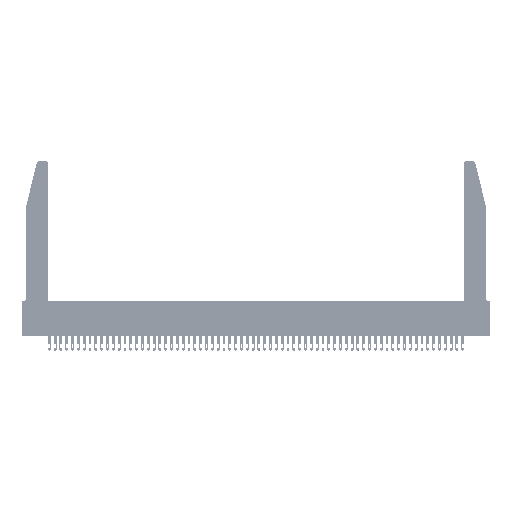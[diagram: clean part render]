
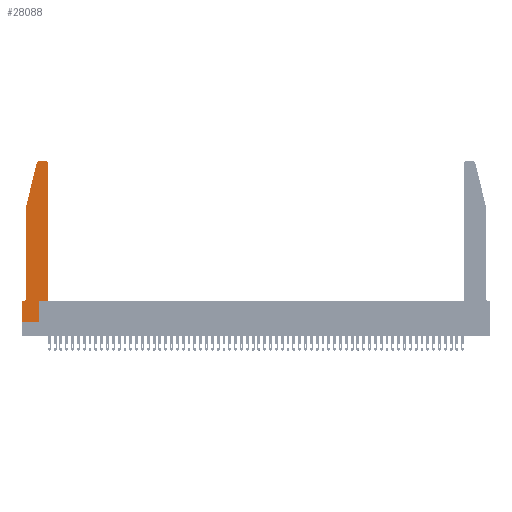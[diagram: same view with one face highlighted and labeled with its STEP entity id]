
A CAD part, top view. The second image highlights one B-rep face of the part: STEP entity #28088.
In plain terms, the highlighted planar face has unit normal (0, 0, 1).
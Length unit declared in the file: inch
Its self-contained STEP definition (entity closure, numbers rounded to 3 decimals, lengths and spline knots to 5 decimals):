
#56 = CARTESIAN_POINT ( 'NONE',  ( 0.0755, 2., 0.37 ) ) ;
#305 = AXIS2_PLACEMENT_3D ( 'NONE', #29494, #3072, #2487 ) ;
#829 = VECTOR ( 'NONE', #48670, 39.37008 ) ;
#1154 = DIRECTION ( 'NONE',  ( 0., -1., 0. ) ) ;
#1818 = AXIS2_PLACEMENT_3D ( 'NONE', #51227, #43113, #55838 ) ;
#1971 = CARTESIAN_POINT ( 'NONE',  ( 0.2605, 2.75, 0.37 ) ) ;
#1988 = VERTEX_POINT ( 'NONE', #7573 ) ;
#2487 = DIRECTION ( 'NONE',  ( -1., 0., 0. ) ) ;
#2605 = LINE ( 'NONE', #44147, #19877 ) ;
#3072 = DIRECTION ( 'NONE',  ( 0., 0., -1. ) ) ;
#5427 = CARTESIAN_POINT ( 'NONE',  ( 0.0755, 2., 0.37 ) ) ;
#7355 = CARTESIAN_POINT ( 'NONE',  ( 0.4205, 2.72, 0.37 ) ) ;
#7429 = EDGE_CURVE ( 'NONE', #29231, #39540, #9327, .T. ) ;
#7573 = CARTESIAN_POINT ( 'NONE',  ( 0.4205, 2.75, 0.37 ) ) ;
#8201 = EDGE_CURVE ( 'NONE', #42058, #14537, #34062, .T. ) ;
#9202 = CIRCLE ( 'NONE', #32443, 0.03 ) ;
#9327 = LINE ( 'NONE', #55491, #31395 ) ;
#11403 = DIRECTION ( 'NONE',  ( 0., 0., 1. ) ) ;
#11597 = EDGE_CURVE ( 'NONE', #39501, #41032, #36417, .T. ) ;
#11616 = CARTESIAN_POINT ( 'NONE',  ( 0.0755, 2., 0.37 ) ) ;
#11705 = DIRECTION ( 'NONE',  ( 0., 1., 0. ) ) ;
#12348 = ORIENTED_EDGE ( 'NONE', *, *, #13615, .T. ) ;
#12365 = ORIENTED_EDGE ( 'NONE', *, *, #8201, .T. ) ;
#12788 = VECTOR ( 'NONE', #28986, 39.37008 ) ;
#13615 = EDGE_CURVE ( 'NONE', #41032, #22787, #20539, .T. ) ;
#14005 = VECTOR ( 'NONE', #20312, 39.37008 ) ;
#14537 = VERTEX_POINT ( 'NONE', #26700 ) ;
#14731 = VERTEX_POINT ( 'NONE', #45286 ) ;
#14789 = CARTESIAN_POINT ( 'NONE',  ( 0.0055, 0.35, 0.37 ) ) ;
#15324 = CARTESIAN_POINT ( 'NONE',  ( 0.284, 2.72, 0.37 ) ) ;
#16478 = ORIENTED_EDGE ( 'NONE', *, *, #24856, .T. ) ;
#16716 = EDGE_CURVE ( 'NONE', #14537, #39501, #16760, .T. ) ;
#16760 = LINE ( 'NONE', #11616, #14005 ) ;
#16932 = EDGE_CURVE ( 'NONE', #27159, #14731, #38811, .T. ) ;
#18839 = CARTESIAN_POINT ( 'NONE',  ( 0.284, 2.75, 0.37 ) ) ;
#19877 = VECTOR ( 'NONE', #47990, 39.37008 ) ;
#20202 = CARTESIAN_POINT ( 'NONE',  ( 0.4505, 0.35, 0.37 ) ) ;
#20312 = DIRECTION ( 'NONE',  ( -0.239, -0.971, 0. ) ) ;
#20539 = CIRCLE ( 'NONE', #305, 0.07 ) ;
#20836 = VECTOR ( 'NONE', #11705, 39.37008 ) ;
#21900 = EDGE_CURVE ( 'NONE', #22787, #27159, #27743, .T. ) ;
#22787 = VERTEX_POINT ( 'NONE', #14789 ) ;
#22901 = EDGE_CURVE ( 'NONE', #55174, #29231, #43647, .T. ) ;
#24856 = EDGE_CURVE ( 'NONE', #14731, #55174, #2605, .T. ) ;
#25391 = DIRECTION ( 'NONE',  ( 0., 1., 0. ) ) ;
#25934 = ORIENTED_EDGE ( 'NONE', *, *, #7429, .T. ) ;
#26446 = EDGE_CURVE ( 'NONE', #39540, #52723, #43712, .T. ) ;
#26700 = CARTESIAN_POINT ( 'NONE',  ( 0.25487, 2.72718, 0.37 ) ) ;
#27159 = VERTEX_POINT ( 'NONE', #41838 ) ;
#27699 = VECTOR ( 'NONE', #25391, 39.37008 ) ;
#27743 = LINE ( 'NONE', #52731, #45721 ) ;
#28088 = ADVANCED_FACE ( 'NONE', ( #46892 ), #47556, .T. ) ;
#28442 = DIRECTION ( 'NONE',  ( 1., 0., 0. ) ) ;
#28839 = DIRECTION ( 'NONE',  ( 1., 0., 0. ) ) ;
#28986 = DIRECTION ( 'NONE',  ( -1., 0., 0. ) ) ;
#29231 = VERTEX_POINT ( 'NONE', #46678 ) ;
#29402 = AXIS2_PLACEMENT_3D ( 'NONE', #15324, #47011, #28839 ) ;
#29494 = CARTESIAN_POINT ( 'NONE',  ( 0.0055, 0.42, 0.37 ) ) ;
#31395 = VECTOR ( 'NONE', #28442, 39.37008 ) ;
#32073 = EDGE_LOOP ( 'NONE', ( #36774, #12365, #33140, #32677, #12348, #38056, #43174, #16478, #46230, #25934, #32912, #44310 ) ) ;
#32443 = AXIS2_PLACEMENT_3D ( 'NONE', #7355, #11403, #56176 ) ;
#32677 = ORIENTED_EDGE ( 'NONE', *, *, #11597, .T. ) ;
#32912 = ORIENTED_EDGE ( 'NONE', *, *, #26446, .T. ) ;
#33140 = ORIENTED_EDGE ( 'NONE', *, *, #16716, .T. ) ;
#33504 = CARTESIAN_POINT ( 'NONE',  ( 0.0755, 0.42, 0.37 ) ) ;
#34062 = CIRCLE ( 'NONE', #29402, 0.03 ) ;
#35086 = EDGE_CURVE ( 'NONE', #1988, #42058, #55605, .T. ) ;
#35550 = CARTESIAN_POINT ( 'NONE',  ( 0., 0., 0.37 ) ) ;
#35964 = EDGE_CURVE ( 'NONE', #52723, #1988, #9202, .T. ) ;
#36417 = LINE ( 'NONE', #5427, #53692 ) ;
#36774 = ORIENTED_EDGE ( 'NONE', *, *, #35086, .T. ) ;
#38056 = ORIENTED_EDGE ( 'NONE', *, *, #21900, .T. ) ;
#38321 = CARTESIAN_POINT ( 'NONE',  ( 0.2865, 0.35, 0.37 ) ) ;
#38811 = LINE ( 'NONE', #35550, #829 ) ;
#39501 = VERTEX_POINT ( 'NONE', #56 ) ;
#39540 = VERTEX_POINT ( 'NONE', #54311 ) ;
#41032 = VERTEX_POINT ( 'NONE', #33504 ) ;
#41838 = CARTESIAN_POINT ( 'NONE',  ( 0., 0.35, 0.37 ) ) ;
#42058 = VERTEX_POINT ( 'NONE', #18839 ) ;
#43113 = DIRECTION ( 'NONE',  ( 0., 0., 1. ) ) ;
#43174 = ORIENTED_EDGE ( 'NONE', *, *, #16932, .T. ) ;
#43647 = LINE ( 'NONE', #38321, #27699 ) ;
#43712 = LINE ( 'NONE', #20202, #20836 ) ;
#44147 = CARTESIAN_POINT ( 'NONE',  ( 0., 0., 0.37 ) ) ;
#44310 = ORIENTED_EDGE ( 'NONE', *, *, #35964, .T. ) ;
#45286 = CARTESIAN_POINT ( 'NONE',  ( 0., 0., 0.37 ) ) ;
#45721 = VECTOR ( 'NONE', #56956, 39.37008 ) ;
#46230 = ORIENTED_EDGE ( 'NONE', *, *, #22901, .T. ) ;
#46678 = CARTESIAN_POINT ( 'NONE',  ( 0.2865, 0.35, 0.37 ) ) ;
#46892 = FACE_OUTER_BOUND ( 'NONE', #32073, .T. ) ;
#47011 = DIRECTION ( 'NONE',  ( 0., 0., 1. ) ) ;
#47556 = PLANE ( 'NONE',  #1818 ) ;
#47990 = DIRECTION ( 'NONE',  ( 1., 0., 0. ) ) ;
#48670 = DIRECTION ( 'NONE',  ( 0., -1., 0. ) ) ;
#50727 = CARTESIAN_POINT ( 'NONE',  ( 0.2865, 0., 0.37 ) ) ;
#51227 = CARTESIAN_POINT ( 'NONE',  ( 0., 0.35, 0.37 ) ) ;
#52347 = CARTESIAN_POINT ( 'NONE',  ( 0.4505, 2.72, 0.37 ) ) ;
#52723 = VERTEX_POINT ( 'NONE', #52347 ) ;
#52731 = CARTESIAN_POINT ( 'NONE',  ( 0.0755, 0.35, 0.37 ) ) ;
#53692 = VECTOR ( 'NONE', #1154, 39.37008 ) ;
#54311 = CARTESIAN_POINT ( 'NONE',  ( 0.4505, 0.35, 0.37 ) ) ;
#55174 = VERTEX_POINT ( 'NONE', #50727 ) ;
#55491 = CARTESIAN_POINT ( 'NONE',  ( 0.4505, 0.35, 0.37 ) ) ;
#55605 = LINE ( 'NONE', #1971, #12788 ) ;
#55838 = DIRECTION ( 'NONE',  ( 1., 0., 0. ) ) ;
#56176 = DIRECTION ( 'NONE',  ( 1., 0., 0. ) ) ;
#56956 = DIRECTION ( 'NONE',  ( -1., 0., 0. ) ) ;
